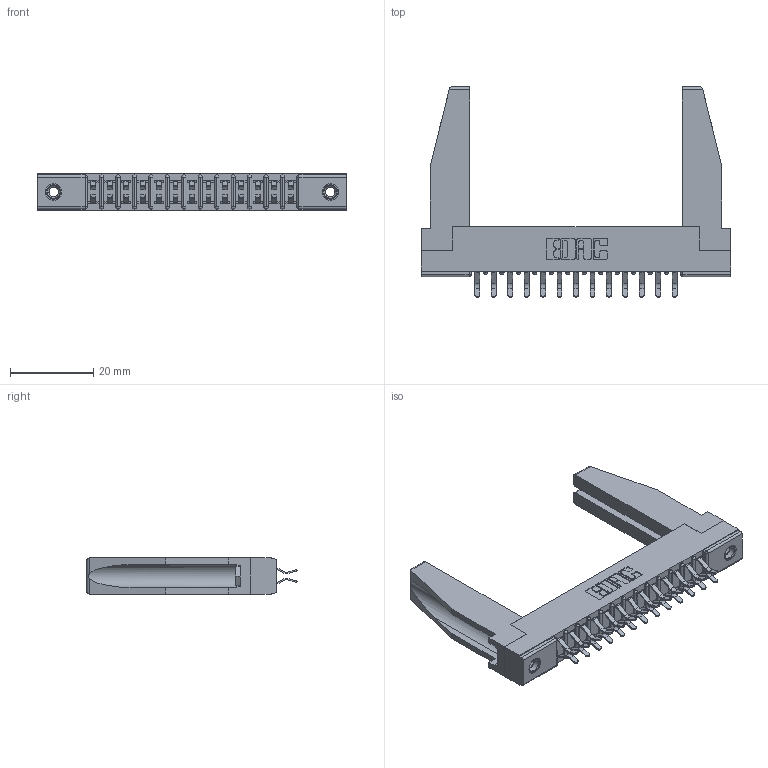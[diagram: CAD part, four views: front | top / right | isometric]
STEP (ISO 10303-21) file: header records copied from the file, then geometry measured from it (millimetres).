
FILE_DESCRIPTION (( 'STEP AP203' ), '1' );
FILE_NAME ('357-026-556-278.STEP', '2019-09-17T23:05:53', ( '' ), ( '' ), 'SwSTEP 2.0', 'SolidWorks 2016', '' );
FILE_SCHEMA (( 'CONFIG_CONTROL_DESIGN' ));
Length unit declared in the file: inch
Products named in the file (5): 307-220-078; 345-250-001_345-250-001-102; 307-290-001_556; 357-026-556-278; 307 Part_.156 Dia Mounting Holes
Assembly tree (31 placements, depth 2):
  357-026-556-278
    307 Part_.156 Dia Mounting Holes
    307-290-001_556  x26
    307-220-078  x2
    345-250-001_345-250-001-102  x2
Bounding box: 74.52 x 50.67 x 8.71 mm (x, y, z)
Volume: 8864.3 mm3; surface area: 11932 mm2
Topology: 31 solids, 31 shells, 1562 faces, 4345 edges, 2814 vertices
Faces by surface type: plane 1012, cylinder 506, sphere 28, cone 12, torus 4
Entity records: 17679 total; most frequent: CARTESIAN_POINT 2911, ORIENTED_EDGE 2840, DIRECTION 2818, EDGE_CURVE 1420, VECTOR 1080, LINE 1080, VERTEX_POINT 920, AXIS2_PLACEMENT_3D 869
